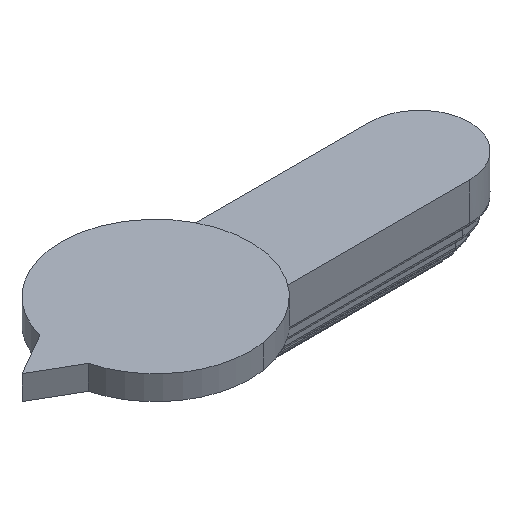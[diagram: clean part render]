
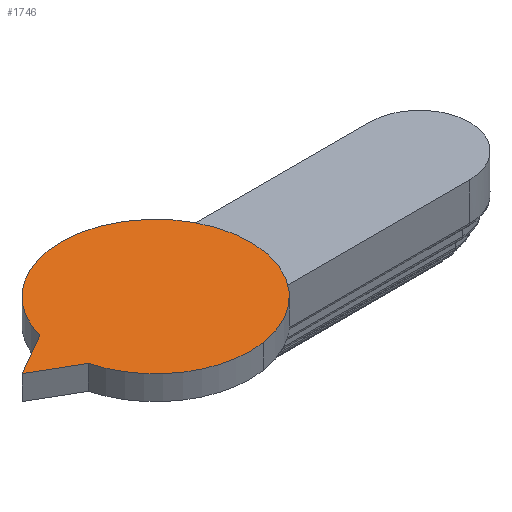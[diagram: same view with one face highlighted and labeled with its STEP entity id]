
A CAD part, isometric view. The second image highlights one B-rep face of the part: STEP entity #1746.
In plain terms, the highlighted planar face has unit normal (0, 0, 1).
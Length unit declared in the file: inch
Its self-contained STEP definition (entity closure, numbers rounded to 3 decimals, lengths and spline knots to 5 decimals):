
#35=CARTESIAN_POINT('',(0.,0.,0.));
#36=DIRECTION('',(0.,0.,1.));
#37=DIRECTION('',(-0.967,-0.256,0.));
#38=AXIS2_PLACEMENT_3D('',#35,#36,#37);
#43=DIRECTION('',(0.866,-0.5,0.));
#44=VECTOR('',#43,0.12237);
#45=CARTESIAN_POINT('',(-0.33675,0.,0.));
#46=LINE('',#45,#44);
#50=DIRECTION('',(-0.866,-0.5,0.));
#51=VECTOR('',#50,0.12237);
#52=CARTESIAN_POINT('',(-0.23078,0.06118,0.));
#53=LINE('',#52,#51);
#57=CARTESIAN_POINT('',(0.,0.,0.));
#58=DIRECTION('',(0.,0.,1.));
#59=DIRECTION('',(-0.667,0.745,0.));
#60=AXIS2_PLACEMENT_3D('',#57,#58,#59);
#65=CARTESIAN_POINT('',(0.,0.,0.));
#66=DIRECTION('',(0.,0.,1.));
#67=DIRECTION('',(-0.148,0.989,0.));
#68=AXIS2_PLACEMENT_3D('',#65,#66,#67);
#73=CARTESIAN_POINT('',(0.,0.,0.));
#74=DIRECTION('',(0.,0.,1.));
#75=DIRECTION('',(0.148,-0.989,0.));
#76=AXIS2_PLACEMENT_3D('',#73,#74,#75);
#81=CARTESIAN_POINT('',(0.,0.,0.));
#82=DIRECTION('',(0.,0.,1.));
#83=DIRECTION('',(-0.549,-0.836,0.));
#84=AXIS2_PLACEMENT_3D('',#81,#82,#83);
#1522=CARTESIAN_POINT('',(0.0353,-0.23613,0.));
#1523=CARTESIAN_POINT('',(-0.0353,0.23613,0.));
#1524=VERTEX_POINT('',#1522);
#1525=VERTEX_POINT('',#1523);
#1692=CARTESIAN_POINT('',(-0.23078,0.06118,0.));
#1693=VERTEX_POINT('',#1692);
#1694=CARTESIAN_POINT('',(-0.15922,0.17791,0.));
#1695=VERTEX_POINT('',#1694);
#1696=CARTESIAN_POINT('',(-0.33675,0.,0.));
#1697=VERTEX_POINT('',#1696);
#1698=CARTESIAN_POINT('',(-0.23078,-0.06118,0.));
#1699=VERTEX_POINT('',#1698);
#1700=CARTESIAN_POINT('',(-0.13116,-0.19949,0.));
#1701=VERTEX_POINT('',#1700);
#1726=CARTESIAN_POINT('',(0.2422,0.24162,0.));
#1727=DIRECTION('',(0.,0.,1.));
#1728=DIRECTION('',(-1.,0.,0.));
#1729=AXIS2_PLACEMENT_3D('',#1726,#1727,#1728);
#1730=PLANE('',#1729);
#1732=ORIENTED_EDGE('',*,*,#1731,.F.);
#1734=ORIENTED_EDGE('',*,*,#1733,.F.);
#1736=ORIENTED_EDGE('',*,*,#1735,.F.);
#1738=ORIENTED_EDGE('',*,*,#1737,.F.);
#1740=ORIENTED_EDGE('',*,*,#1739,.F.);
#1741=ORIENTED_EDGE('',*,*,#1707,.F.);
#1743=ORIENTED_EDGE('',*,*,#1742,.F.);
#1744=EDGE_LOOP('',(#1732,#1734,#1736,#1738,#1740,#1741,#1743));
#1745=FACE_OUTER_BOUND('',#1744,.F.);
#39=CIRCLE('',#38,0.23875);
#61=CIRCLE('',#60,0.23875);
#69=CIRCLE('',#68,0.23875);
#77=CIRCLE('',#76,0.23875);
#85=CIRCLE('',#84,0.23875);
#1707=EDGE_CURVE('',#1524,#1525,#77,.T.);
#1731=EDGE_CURVE('',#1699,#1701,#39,.T.);
#1733=EDGE_CURVE('',#1697,#1699,#46,.T.);
#1735=EDGE_CURVE('',#1693,#1697,#53,.T.);
#1737=EDGE_CURVE('',#1695,#1693,#61,.T.);
#1739=EDGE_CURVE('',#1525,#1695,#69,.T.);
#1742=EDGE_CURVE('',#1701,#1524,#85,.T.);
#1746=ADVANCED_FACE('',(#1745),#1730,.T.);
